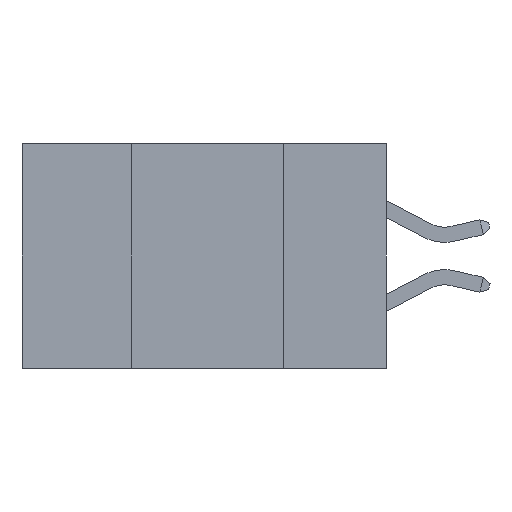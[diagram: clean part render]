
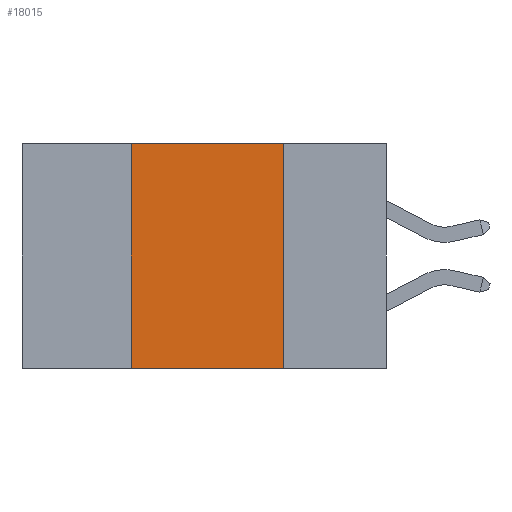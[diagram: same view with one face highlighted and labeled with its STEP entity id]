
A CAD part, left-side view. The second image highlights one B-rep face of the part: STEP entity #18015.
In plain terms, the highlighted planar face has unit normal (-1, 0, 0).
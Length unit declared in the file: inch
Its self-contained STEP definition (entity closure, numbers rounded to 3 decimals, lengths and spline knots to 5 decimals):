
#1035 = VECTOR ( 'NONE', #9566, 39.37008 ) ;
#1709 = DIRECTION ( 'NONE',  ( 0., 0., -1. ) ) ;
#2095 = CARTESIAN_POINT ( 'NONE',  ( 0., 0.42, -0.37 ) ) ;
#2299 = LINE ( 'NONE', #8851, #12096 ) ;
#5279 = VERTEX_POINT ( 'NONE', #2095 ) ;
#6093 = VECTOR ( 'NONE', #20208, 39.37008 ) ;
#6141 = EDGE_CURVE ( 'NONE', #5279, #20088, #14351, .T. ) ;
#6336 = EDGE_LOOP ( 'NONE', ( #11543, #7482, #8563, #13129 ) ) ;
#7320 = EDGE_CURVE ( 'NONE', #5279, #17350, #16475, .T. ) ;
#7482 = ORIENTED_EDGE ( 'NONE', *, *, #8474, .F. ) ;
#8195 = CARTESIAN_POINT ( 'NONE',  ( 0., 0.17, -0.37 ) ) ;
#8474 = EDGE_CURVE ( 'NONE', #17350, #22143, #2299, .T. ) ;
#8563 = ORIENTED_EDGE ( 'NONE', *, *, #7320, .F. ) ;
#8851 = CARTESIAN_POINT ( 'NONE',  ( 0., 0.6, 0. ) ) ;
#9566 = DIRECTION ( 'NONE',  ( 0., -1., 0. ) ) ;
#9651 = EDGE_CURVE ( 'NONE', #22143, #20088, #19824, .T. ) ;
#10330 = PLANE ( 'NONE',  #14587 ) ;
#11364 = VECTOR ( 'NONE', #18052, 39.37008 ) ;
#11543 = ORIENTED_EDGE ( 'NONE', *, *, #9651, .F. ) ;
#12096 = VECTOR ( 'NONE', #19111, 39.37008 ) ;
#12126 = DIRECTION ( 'NONE',  ( 1., 0., 0. ) ) ;
#12952 = CARTESIAN_POINT ( 'NONE',  ( 0., 0.17, -0.37 ) ) ;
#13129 = ORIENTED_EDGE ( 'NONE', *, *, #6141, .T. ) ;
#14351 = LINE ( 'NONE', #21546, #1035 ) ;
#14587 = AXIS2_PLACEMENT_3D ( 'NONE', #22401, #12126, #1709 ) ;
#14935 = FACE_OUTER_BOUND ( 'NONE', #6336, .T. ) ;
#16475 = LINE ( 'NONE', #17976, #11364 ) ;
#16514 = CARTESIAN_POINT ( 'NONE',  ( 0., 0.17, 0. ) ) ;
#17342 = CARTESIAN_POINT ( 'NONE',  ( 0., 0.42, 0. ) ) ;
#17350 = VERTEX_POINT ( 'NONE', #17342 ) ;
#17976 = CARTESIAN_POINT ( 'NONE',  ( 0., 0.42, -0.37 ) ) ;
#18015 = ADVANCED_FACE ( 'NONE', ( #14935 ), #10330, .F. ) ;
#18052 = DIRECTION ( 'NONE',  ( 0., 0., 1. ) ) ;
#19111 = DIRECTION ( 'NONE',  ( 0., -1., 0. ) ) ;
#19824 = LINE ( 'NONE', #8195, #6093 ) ;
#20088 = VERTEX_POINT ( 'NONE', #12952 ) ;
#20208 = DIRECTION ( 'NONE',  ( 0., 0., -1. ) ) ;
#21546 = CARTESIAN_POINT ( 'NONE',  ( 0., 0.6, -0.37 ) ) ;
#22143 = VERTEX_POINT ( 'NONE', #16514 ) ;
#22401 = CARTESIAN_POINT ( 'NONE',  ( 0., 0.6, 0. ) ) ;
